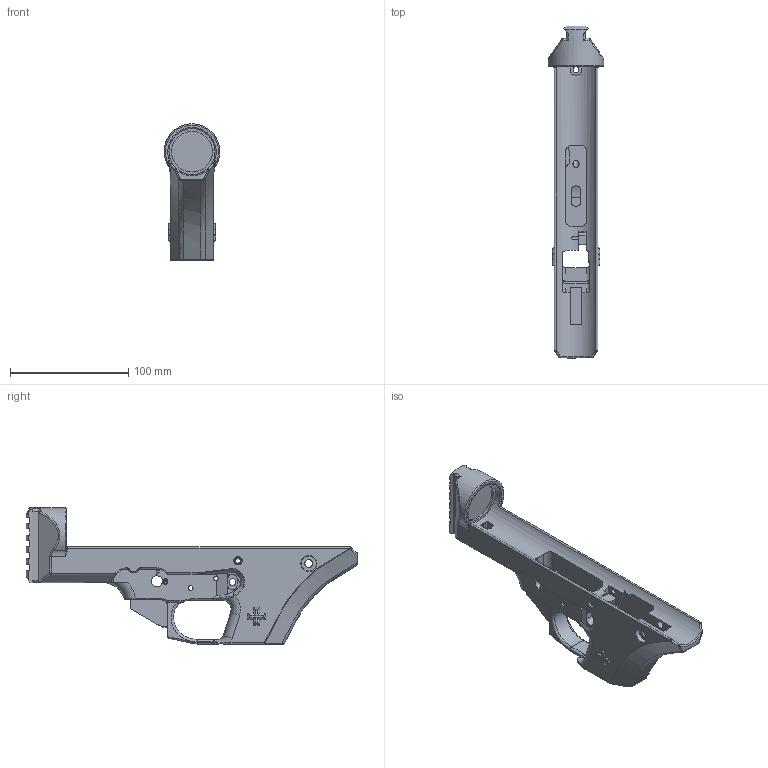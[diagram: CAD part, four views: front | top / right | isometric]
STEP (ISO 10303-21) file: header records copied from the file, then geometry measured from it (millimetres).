
FILE_DESCRIPTION(/* description */ (''),/* implementation_level */ '2;1');
FILE_NAME(/* name */ 'GlockReciever v52.step',/* time_stamp */ '2022-08-23T17:48:52-04:00',/* author */ (''),/* organization */ (''),/* preprocessor_version */ 'ST-DEVELOPER v19',/* originating_system */ 'Autodesk Translation Framework v11.7.0.108',/* authorisation */ '');
FILE_SCHEMA (('AUTOMOTIVE_DESIGN { 1 0 10303 214 3 1 1 }'));
Length unit declared in the file: millimetre
Products named in the file (1): GlockReciever
Bounding box: 46.98 x 280.74 x 115.2 mm (x, y, z)
Volume: 279096.7 mm3; surface area: 76281.8 mm2
Topology: 1 solids, 1 shells, 530 faces, 1442 edges, 911 vertices
Faces by surface type: plane 181, cylinder 169, bspline 121, torus 42, sphere 14, cone 3
Full cylindrical faces by diameter (mm): 1.75 x2, 3.75 x1, 4 x5, 4.2 x2, 5 x1, 5.2 x1, 5.8 x1, 6 x2, 6.5 x2, 8.5 x1, 9.5 x3, 12.7 x2, 34.4 x1, 39 x1
Entity records: 22641 total; most frequent: CARTESIAN_POINT 9888, ORIENTED_EDGE 2868, DIRECTION 2376, EDGE_CURVE 1434, VERTEX_POINT 911, AXIS2_PLACEMENT_3D 855, LINE 666, VECTOR 666
